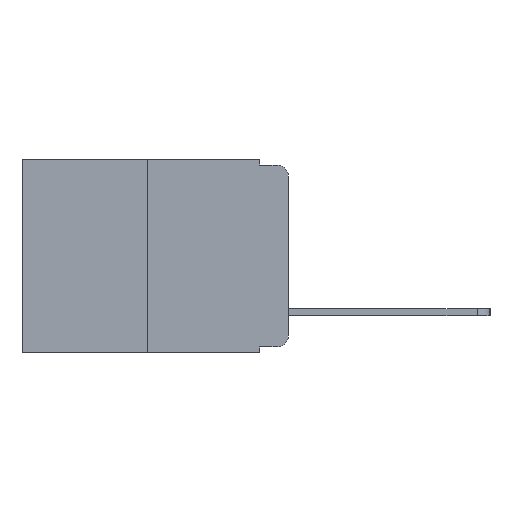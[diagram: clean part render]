
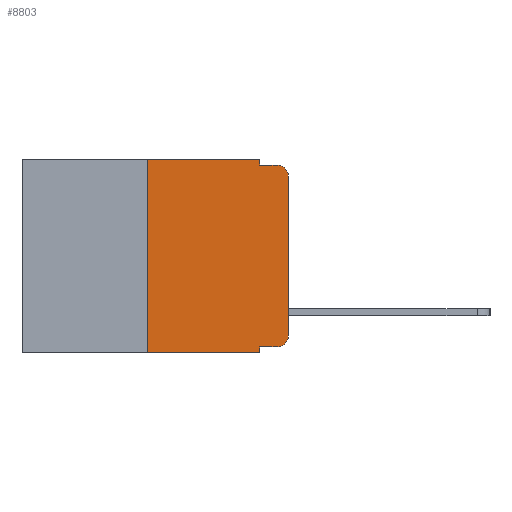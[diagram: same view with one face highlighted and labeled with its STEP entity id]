
A CAD part, left-side view. The second image highlights one B-rep face of the part: STEP entity #8803.
In plain terms, the highlighted planar face has unit normal (-1, 0, 0).
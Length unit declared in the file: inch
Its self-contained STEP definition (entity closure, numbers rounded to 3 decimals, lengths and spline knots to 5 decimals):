
#87 = ORIENTED_EDGE ( 'NONE', *, *, #4961, .T. ) ;
#301 = ORIENTED_EDGE ( 'NONE', *, *, #1204, .T. ) ;
#493 = LINE ( 'NONE', #7478, #4219 ) ;
#1204 = EDGE_CURVE ( 'NONE', #9067, #5418, #493, .T. ) ;
#1282 = LINE ( 'NONE', #3629, #4890 ) ;
#1471 = CARTESIAN_POINT ( 'NONE',  ( 0., 0.02, -0.313 ) ) ;
#1539 = LINE ( 'NONE', #8632, #14829 ) ;
#2009 = VERTEX_POINT ( 'NONE', #4843 ) ;
#2517 = DIRECTION ( 'NONE',  ( 0., -1., 0. ) ) ;
#2639 = DIRECTION ( 'NONE',  ( 0., 0., -1. ) ) ;
#2919 = DIRECTION ( 'NONE',  ( 0., 0., -1. ) ) ;
#3044 = CARTESIAN_POINT ( 'NONE',  ( 0., 0.051, 0. ) ) ;
#3311 = CARTESIAN_POINT ( 'NONE',  ( 0., 0.051, -0.01 ) ) ;
#3345 = ORIENTED_EDGE ( 'NONE', *, *, #11797, .F. ) ;
#3629 = CARTESIAN_POINT ( 'NONE',  ( 0., 0.473, -0.343 ) ) ;
#3935 = CARTESIAN_POINT ( 'NONE',  ( 0., 0.473, 0. ) ) ;
#4079 = VERTEX_POINT ( 'NONE', #3311 ) ;
#4219 = VECTOR ( 'NONE', #6140, 39.37008 ) ;
#4353 = ORIENTED_EDGE ( 'NONE', *, *, #10113, .F. ) ;
#4399 = DIRECTION ( 'NONE',  ( -1., 0., 0. ) ) ;
#4600 = LINE ( 'NONE', #3935, #14375 ) ;
#4643 = VECTOR ( 'NONE', #12152, 39.37008 ) ;
#4663 = ORIENTED_EDGE ( 'NONE', *, *, #13451, .T. ) ;
#4679 = CARTESIAN_POINT ( 'NONE',  ( 0., 0.25, -0.343 ) ) ;
#4720 = DIRECTION ( 'NONE',  ( 0., 0., 1. ) ) ;
#4843 = CARTESIAN_POINT ( 'NONE',  ( 0., 0.051, -0.343 ) ) ;
#4890 = VECTOR ( 'NONE', #2517, 39.37008 ) ;
#4928 = LINE ( 'NONE', #8997, #11435 ) ;
#4961 = EDGE_CURVE ( 'NONE', #12874, #2009, #1282, .T. ) ;
#5123 = AXIS2_PLACEMENT_3D ( 'NONE', #12139, #4399, #13377 ) ;
#5198 = DIRECTION ( 'NONE',  ( 0., -1., 0. ) ) ;
#5418 = VERTEX_POINT ( 'NONE', #7180 ) ;
#5780 = ORIENTED_EDGE ( 'NONE', *, *, #6641, .F. ) ;
#6104 = DIRECTION ( 'NONE',  ( 1., 0., 0. ) ) ;
#6140 = DIRECTION ( 'NONE',  ( 0., -1., 0. ) ) ;
#6518 = CIRCLE ( 'NONE', #11238, 0.02 ) ;
#6641 = EDGE_CURVE ( 'NONE', #9067, #2009, #14769, .T. ) ;
#6667 = FACE_OUTER_BOUND ( 'NONE', #16493, .T. ) ;
#7180 = CARTESIAN_POINT ( 'NONE',  ( 0., 0.02, -0.333 ) ) ;
#7207 = ORIENTED_EDGE ( 'NONE', *, *, #16457, .T. ) ;
#7461 = VERTEX_POINT ( 'NONE', #13914 ) ;
#7478 = CARTESIAN_POINT ( 'NONE',  ( 0., 0.051, -0.333 ) ) ;
#8229 = DIRECTION ( 'NONE',  ( 0., -1., 0. ) ) ;
#8553 = EDGE_CURVE ( 'NONE', #15155, #14963, #4600, .T. ) ;
#8632 = CARTESIAN_POINT ( 'NONE',  ( 0., 0., 0. ) ) ;
#8674 = VECTOR ( 'NONE', #8229, 39.37008 ) ;
#8711 = CARTESIAN_POINT ( 'NONE',  ( 0., 0.473, 0. ) ) ;
#8803 = ADVANCED_FACE ( 'NONE', ( #6667 ), #12516, .F. ) ;
#8981 = ORIENTED_EDGE ( 'NONE', *, *, #15039, .T. ) ;
#8997 = CARTESIAN_POINT ( 'NONE',  ( 0., 0.25, 0. ) ) ;
#9067 = VERTEX_POINT ( 'NONE', #14323 ) ;
#9114 = ORIENTED_EDGE ( 'NONE', *, *, #10964, .F. ) ;
#9194 = CARTESIAN_POINT ( 'NONE',  ( 0., 0.051, 0. ) ) ;
#9195 = CARTESIAN_POINT ( 'NONE',  ( 0., 0., -0.03 ) ) ;
#9523 = CARTESIAN_POINT ( 'NONE',  ( 0., 0.051, -0.01 ) ) ;
#9597 = VERTEX_POINT ( 'NONE', #9195 ) ;
#10113 = EDGE_CURVE ( 'NONE', #12874, #15155, #4928, .T. ) ;
#10200 = CARTESIAN_POINT ( 'NONE',  ( 0., 0.25, 0. ) ) ;
#10733 = DIRECTION ( 'NONE',  ( -1., 0., 0. ) ) ;
#10964 = EDGE_CURVE ( 'NONE', #14963, #4079, #15306, .T. ) ;
#11238 = AXIS2_PLACEMENT_3D ( 'NONE', #1471, #10733, #2919 ) ;
#11413 = CIRCLE ( 'NONE', #5123, 0.02 ) ;
#11435 = VECTOR ( 'NONE', #16383, 39.37008 ) ;
#11439 = AXIS2_PLACEMENT_3D ( 'NONE', #8711, #6104, #14934 ) ;
#11797 = EDGE_CURVE ( 'NONE', #4079, #7461, #15273, .T. ) ;
#12105 = VECTOR ( 'NONE', #2639, 39.37008 ) ;
#12139 = CARTESIAN_POINT ( 'NONE',  ( 0., 0.02, -0.03 ) ) ;
#12152 = DIRECTION ( 'NONE',  ( 0., 0., -1. ) ) ;
#12153 = CARTESIAN_POINT ( 'NONE',  ( 0., 0., -0.313 ) ) ;
#12516 = PLANE ( 'NONE',  #11439 ) ;
#12874 = VERTEX_POINT ( 'NONE', #4679 ) ;
#13377 = DIRECTION ( 'NONE',  ( 0., 0., -1. ) ) ;
#13451 = EDGE_CURVE ( 'NONE', #9597, #7461, #11413, .T. ) ;
#13914 = CARTESIAN_POINT ( 'NONE',  ( 0., 0.02, -0.01 ) ) ;
#14072 = ORIENTED_EDGE ( 'NONE', *, *, #8553, .F. ) ;
#14281 = VERTEX_POINT ( 'NONE', #12153 ) ;
#14323 = CARTESIAN_POINT ( 'NONE',  ( 0., 0.051, -0.333 ) ) ;
#14375 = VECTOR ( 'NONE', #5198, 39.37008 ) ;
#14470 = CARTESIAN_POINT ( 'NONE',  ( 0., 0.051, 0. ) ) ;
#14769 = LINE ( 'NONE', #3044, #4643 ) ;
#14829 = VECTOR ( 'NONE', #4720, 39.37008 ) ;
#14934 = DIRECTION ( 'NONE',  ( 0., 0., -1. ) ) ;
#14963 = VERTEX_POINT ( 'NONE', #14470 ) ;
#15039 = EDGE_CURVE ( 'NONE', #14281, #9597, #1539, .T. ) ;
#15155 = VERTEX_POINT ( 'NONE', #10200 ) ;
#15273 = LINE ( 'NONE', #9523, #8674 ) ;
#15306 = LINE ( 'NONE', #9194, #12105 ) ;
#16383 = DIRECTION ( 'NONE',  ( 0., 0., 1. ) ) ;
#16457 = EDGE_CURVE ( 'NONE', #5418, #14281, #6518, .T. ) ;
#16493 = EDGE_LOOP ( 'NONE', ( #8981, #4663, #3345, #9114, #14072, #4353, #87, #5780, #301, #7207 ) ) ;
